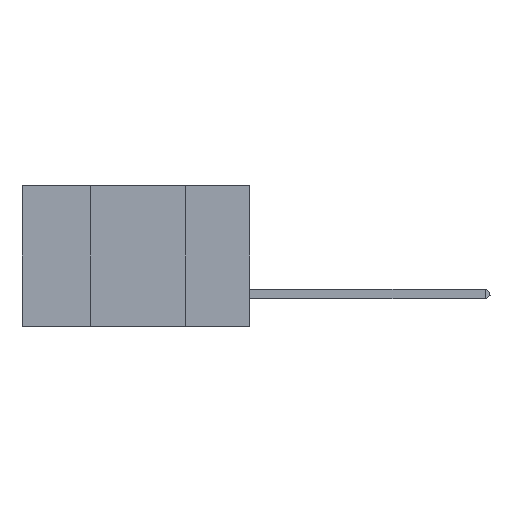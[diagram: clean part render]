
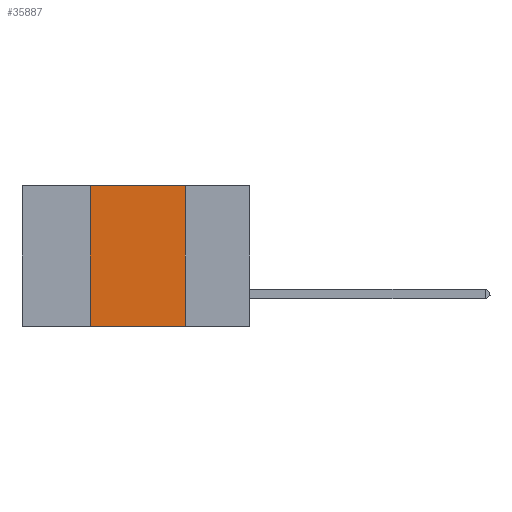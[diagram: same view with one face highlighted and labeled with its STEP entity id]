
A CAD part, left-side view. The second image highlights one B-rep face of the part: STEP entity #35887.
In plain terms, the highlighted planar face has unit normal (-1, 0, 0).
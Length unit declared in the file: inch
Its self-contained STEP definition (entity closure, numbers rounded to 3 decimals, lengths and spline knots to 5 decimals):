
#807 = VERTEX_POINT ( 'NONE', #18923 ) ;
#2924 = PLANE ( 'NONE',  #21259 ) ;
#3947 = CARTESIAN_POINT ( 'NONE',  ( 0., 0.6, 0. ) ) ;
#4120 = VERTEX_POINT ( 'NONE', #32655 ) ;
#5432 = VERTEX_POINT ( 'NONE', #30824 ) ;
#6131 = DIRECTION ( 'NONE',  ( 0., -1., 0. ) ) ;
#11373 = EDGE_LOOP ( 'NONE', ( #27190, #17741, #43189, #32612 ) ) ;
#11486 = EDGE_CURVE ( 'NONE', #4120, #31841, #25753, .T. ) ;
#15938 = VECTOR ( 'NONE', #18872, 39.37008 ) ;
#16466 = DIRECTION ( 'NONE',  ( 0., 0., 1. ) ) ;
#17284 = CARTESIAN_POINT ( 'NONE',  ( 0., 0.6, -0.37 ) ) ;
#17615 = LINE ( 'NONE', #38760, #18168 ) ;
#17741 = ORIENTED_EDGE ( 'NONE', *, *, #11486, .F. ) ;
#18168 = VECTOR ( 'NONE', #16466, 39.37008 ) ;
#18872 = DIRECTION ( 'NONE',  ( 0., -1., 0. ) ) ;
#18923 = CARTESIAN_POINT ( 'NONE',  ( 0., 0.17, -0.37 ) ) ;
#20228 = LINE ( 'NONE', #23963, #26518 ) ;
#21106 = CARTESIAN_POINT ( 'NONE',  ( 0., 0.6, 0. ) ) ;
#21259 = AXIS2_PLACEMENT_3D ( 'NONE', #21106, #32346, #39826 ) ;
#23890 = FACE_OUTER_BOUND ( 'NONE', #11373, .T. ) ;
#23963 = CARTESIAN_POINT ( 'NONE',  ( 0., 0.17, 0. ) ) ;
#25753 = LINE ( 'NONE', #3947, #15938 ) ;
#26518 = VECTOR ( 'NONE', #27339, 39.37008 ) ;
#27190 = ORIENTED_EDGE ( 'NONE', *, *, #45740, .F. ) ;
#27339 = DIRECTION ( 'NONE',  ( 0., 0., -1. ) ) ;
#28440 = LINE ( 'NONE', #17284, #33583 ) ;
#28894 = EDGE_CURVE ( 'NONE', #5432, #807, #28440, .T. ) ;
#30824 = CARTESIAN_POINT ( 'NONE',  ( 0., 0.42, -0.37 ) ) ;
#31841 = VERTEX_POINT ( 'NONE', #47969 ) ;
#32104 = EDGE_CURVE ( 'NONE', #5432, #4120, #17615, .T. ) ;
#32346 = DIRECTION ( 'NONE',  ( 1., 0., 0. ) ) ;
#32612 = ORIENTED_EDGE ( 'NONE', *, *, #28894, .T. ) ;
#32655 = CARTESIAN_POINT ( 'NONE',  ( 0., 0.42, 0. ) ) ;
#33583 = VECTOR ( 'NONE', #6131, 39.37008 ) ;
#35887 = ADVANCED_FACE ( 'NONE', ( #23890 ), #2924, .F. ) ;
#38760 = CARTESIAN_POINT ( 'NONE',  ( 0., 0.42, 0. ) ) ;
#39826 = DIRECTION ( 'NONE',  ( 0., 0., -1. ) ) ;
#43189 = ORIENTED_EDGE ( 'NONE', *, *, #32104, .F. ) ;
#45740 = EDGE_CURVE ( 'NONE', #31841, #807, #20228, .T. ) ;
#47969 = CARTESIAN_POINT ( 'NONE',  ( 0., 0.17, 0. ) ) ;
